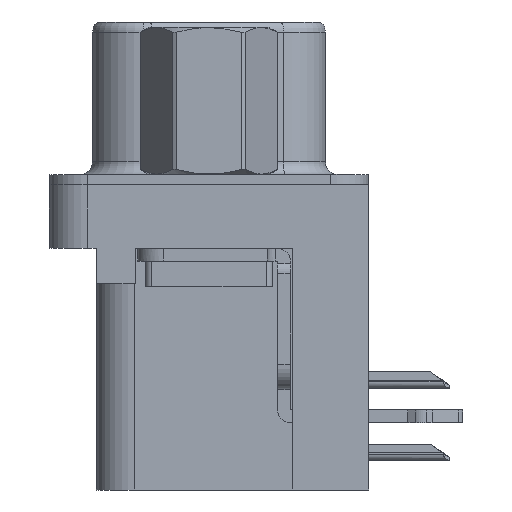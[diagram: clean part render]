
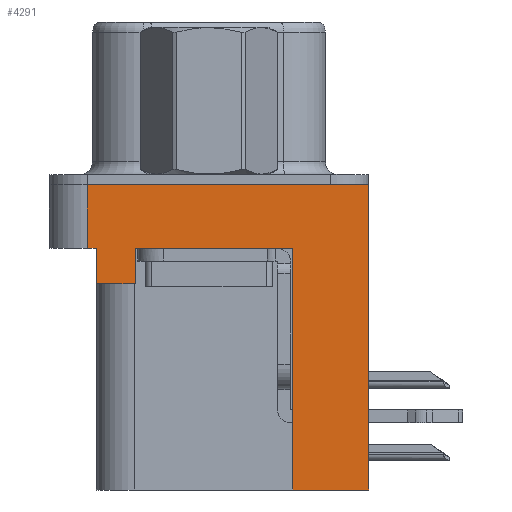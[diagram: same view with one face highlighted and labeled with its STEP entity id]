
A CAD part, left-side view. The second image highlights one B-rep face of the part: STEP entity #4291.
In plain terms, the highlighted planar face has unit normal (-1, 0, 0).
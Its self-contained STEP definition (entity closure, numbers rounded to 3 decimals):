
#393 = DIRECTION ( 'NONE',  ( 0., -1., 0. ) ) ;
#936 = VERTEX_POINT ( 'NONE', #28620 ) ;
#1652 = DIRECTION ( 'NONE',  ( 0., 0., 1. ) ) ;
#1719 = DIRECTION ( 'NONE',  ( 0., 0., 1. ) ) ;
#2938 = ORIENTED_EDGE ( 'NONE', *, *, #21263, .T. ) ;
#3106 = CARTESIAN_POINT ( 'NONE',  ( -2.91, 4.425, -2.5 ) ) ;
#3544 = CARTESIAN_POINT ( 'NONE',  ( -2.91, -6.275, -2.5 ) ) ;
#4088 = ORIENTED_EDGE ( 'NONE', *, *, #29070, .T. ) ;
#4253 = LINE ( 'NONE', #13184, #14406 ) ;
#4291 = ADVANCED_FACE ( 'NONE', ( #15440 ), #11954, .T. ) ;
#5151 = CARTESIAN_POINT ( 'NONE',  ( -2.91, -3.295, -2.5 ) ) ;
#5202 = CARTESIAN_POINT ( 'NONE',  ( -2.91, -6.275, -2.5 ) ) ;
#5461 = DIRECTION ( 'NONE',  ( 0., 1., 0. ) ) ;
#5761 = LINE ( 'NONE', #15463, #13571 ) ;
#6284 = LINE ( 'NONE', #26832, #20660 ) ;
#6710 = VERTEX_POINT ( 'NONE', #17171 ) ;
#7261 = EDGE_CURVE ( 'NONE', #22831, #22082, #6284, .T. ) ;
#7267 = CARTESIAN_POINT ( 'NONE',  ( -2.91, 2.895, -2.5 ) ) ;
#7543 = CARTESIAN_POINT ( 'NONE',  ( -2.91, 2.895, -3.9 ) ) ;
#8525 = VECTOR ( 'NONE', #24322, 1000. ) ;
#8863 = EDGE_CURVE ( 'NONE', #27836, #30190, #5761, .T. ) ;
#9302 = LINE ( 'NONE', #22489, #18564 ) ;
#9871 = LINE ( 'NONE', #22520, #23495 ) ;
#9941 = ORIENTED_EDGE ( 'NONE', *, *, #26176, .F. ) ;
#10579 = ORIENTED_EDGE ( 'NONE', *, *, #31813, .T. ) ;
#10584 = LINE ( 'NONE', #5202, #29352 ) ;
#11954 = PLANE ( 'NONE',  #13871 ) ;
#12230 = VERTEX_POINT ( 'NONE', #25714 ) ;
#12597 = ORIENTED_EDGE ( 'NONE', *, *, #7261, .F. ) ;
#13017 = EDGE_CURVE ( 'NONE', #24807, #31298, #29125, .T. ) ;
#13184 = CARTESIAN_POINT ( 'NONE',  ( -2.91, -6.275, 0. ) ) ;
#13274 = DIRECTION ( 'NONE',  ( 0., 0., 1. ) ) ;
#13548 = VECTOR ( 'NONE', #18868, 1000. ) ;
#13571 = VECTOR ( 'NONE', #13274, 1000. ) ;
#13871 = AXIS2_PLACEMENT_3D ( 'NONE', #14061, #16536, #1719 ) ;
#14061 = CARTESIAN_POINT ( 'NONE',  ( -2.91, -6.275, -2.5 ) ) ;
#14406 = VECTOR ( 'NONE', #393, 1000. ) ;
#15172 = CARTESIAN_POINT ( 'NONE',  ( -2.91, 2.895, -3.9 ) ) ;
#15440 = FACE_OUTER_BOUND ( 'NONE', #24902, .T. ) ;
#15463 = CARTESIAN_POINT ( 'NONE',  ( -2.91, 4.425, -3.9 ) ) ;
#16536 = DIRECTION ( 'NONE',  ( -1., 0., 0. ) ) ;
#16901 = VERTEX_POINT ( 'NONE', #20348 ) ;
#16953 = ORIENTED_EDGE ( 'NONE', *, *, #27179, .F. ) ;
#17135 = CARTESIAN_POINT ( 'NONE',  ( -2.91, -3.295, -12. ) ) ;
#17171 = CARTESIAN_POINT ( 'NONE',  ( -2.91, -6.275, -12. ) ) ;
#17350 = EDGE_CURVE ( 'NONE', #24807, #27836, #9871, .T. ) ;
#18564 = VECTOR ( 'NONE', #27212, 1000. ) ;
#18868 = DIRECTION ( 'NONE',  ( 0., 0., 1. ) ) ;
#20348 = CARTESIAN_POINT ( 'NONE',  ( -2.91, -6.275, 0. ) ) ;
#20660 = VECTOR ( 'NONE', #1652, 1000. ) ;
#21263 = EDGE_CURVE ( 'NONE', #12230, #30190, #23073, .T. ) ;
#22082 = VERTEX_POINT ( 'NONE', #5151 ) ;
#22235 = DIRECTION ( 'NONE',  ( 0., -1., 0. ) ) ;
#22489 = CARTESIAN_POINT ( 'NONE',  ( -2.91, 4.775, -2.5 ) ) ;
#22520 = CARTESIAN_POINT ( 'NONE',  ( -2.91, 4.425, -3.9 ) ) ;
#22831 = VERTEX_POINT ( 'NONE', #30882 ) ;
#23073 = LINE ( 'NONE', #28899, #23863 ) ;
#23355 = ORIENTED_EDGE ( 'NONE', *, *, #13017, .T. ) ;
#23495 = VECTOR ( 'NONE', #5461, 1000. ) ;
#23777 = DIRECTION ( 'NONE',  ( 0., 0., 1. ) ) ;
#23863 = VECTOR ( 'NONE', #26813, 1000. ) ;
#24322 = DIRECTION ( 'NONE',  ( 0., 1., 0. ) ) ;
#24807 = VERTEX_POINT ( 'NONE', #15172 ) ;
#24902 = EDGE_LOOP ( 'NONE', ( #16953, #31863, #2938, #25783, #26115, #23355, #10579, #12597, #9941, #4088 ) ) ;
#25697 = CARTESIAN_POINT ( 'NONE',  ( -2.91, 4.425, -3.9 ) ) ;
#25714 = CARTESIAN_POINT ( 'NONE',  ( -2.91, 4.775, -2.5 ) ) ;
#25783 = ORIENTED_EDGE ( 'NONE', *, *, #8863, .F. ) ;
#25923 = EDGE_CURVE ( 'NONE', #12230, #936, #9302, .T. ) ;
#26115 = ORIENTED_EDGE ( 'NONE', *, *, #17350, .F. ) ;
#26176 = EDGE_CURVE ( 'NONE', #6710, #22831, #31894, .T. ) ;
#26813 = DIRECTION ( 'NONE',  ( 0., -1., 0. ) ) ;
#26832 = CARTESIAN_POINT ( 'NONE',  ( -2.91, -3.295, -12. ) ) ;
#27002 = VECTOR ( 'NONE', #23777, 1000. ) ;
#27179 = EDGE_CURVE ( 'NONE', #936, #16901, #4253, .T. ) ;
#27212 = DIRECTION ( 'NONE',  ( 0., 0., 1. ) ) ;
#27836 = VERTEX_POINT ( 'NONE', #25697 ) ;
#28125 = LINE ( 'NONE', #3544, #27002 ) ;
#28620 = CARTESIAN_POINT ( 'NONE',  ( -2.91, 4.775, 0. ) ) ;
#28899 = CARTESIAN_POINT ( 'NONE',  ( -2.91, -6.275, -2.5 ) ) ;
#29070 = EDGE_CURVE ( 'NONE', #6710, #16901, #28125, .T. ) ;
#29125 = LINE ( 'NONE', #7543, #13548 ) ;
#29352 = VECTOR ( 'NONE', #22235, 1000. ) ;
#30190 = VERTEX_POINT ( 'NONE', #3106 ) ;
#30882 = CARTESIAN_POINT ( 'NONE',  ( -2.91, -3.295, -12. ) ) ;
#31298 = VERTEX_POINT ( 'NONE', #7267 ) ;
#31813 = EDGE_CURVE ( 'NONE', #31298, #22082, #10584, .T. ) ;
#31863 = ORIENTED_EDGE ( 'NONE', *, *, #25923, .F. ) ;
#31894 = LINE ( 'NONE', #17135, #8525 ) ;
